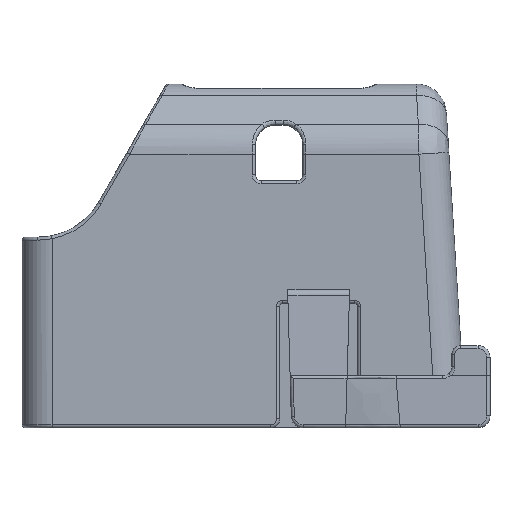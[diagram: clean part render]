
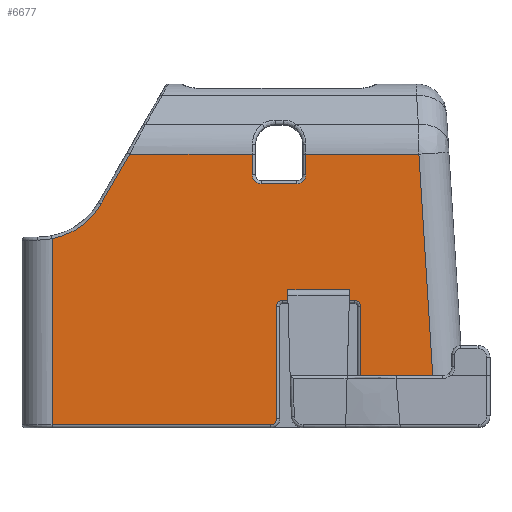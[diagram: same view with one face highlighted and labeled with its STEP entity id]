
A CAD part, left-side view. The second image highlights one B-rep face of the part: STEP entity #6677.
In plain terms, the highlighted planar face has unit normal (-1, 0, 0).
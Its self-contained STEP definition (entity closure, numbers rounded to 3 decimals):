
#21=PLANE('',#7149);
#565=LINE('',#10031,#1024);
#567=LINE('',#10138,#1026);
#568=LINE('',#10146,#1027);
#572=LINE('',#10219,#1031);
#573=LINE('',#10221,#1032);
#574=LINE('',#10225,#1033);
#575=LINE('',#10227,#1034);
#576=LINE('',#10231,#1035);
#577=LINE('',#10235,#1036);
#578=LINE('',#10237,#1037);
#579=LINE('',#10239,#1038);
#580=LINE('',#10241,#1039);
#581=LINE('',#10243,#1040);
#582=LINE('',#10247,#1041);
#583=LINE('',#10251,#1042);
#584=LINE('',#10253,#1043);
#585=LINE('',#10254,#1044);
#1024=VECTOR('',#7941,10.);
#1026=VECTOR('',#7969,10.);
#1027=VECTOR('',#7980,10.);
#1031=VECTOR('',#8000,10.);
#1032=VECTOR('',#8001,10.);
#1033=VECTOR('',#8004,10.);
#1034=VECTOR('',#8005,10.);
#1035=VECTOR('',#8008,10.);
#1036=VECTOR('',#8011,10.);
#1037=VECTOR('',#8012,10.);
#1038=VECTOR('',#8013,10.);
#1039=VECTOR('',#8014,10.);
#1040=VECTOR('',#8015,0.5);
#1041=VECTOR('',#8018,10.);
#1042=VECTOR('',#8021,10.);
#1043=VECTOR('',#8022,10.);
#1044=VECTOR('',#8023,10.);
#1631=FACE_OUTER_BOUND('',#2044,.T.);
#2044=EDGE_LOOP('',(#4598,#4599,#4600,#4601,#4602,#4603,#4604,#4605,#4606,
#4607,#4608,#4609,#4610,#4611,#4612,#4613,#4614,#4615,#4616,#4617,#4618,
#4619,#4620,#4621));
#2453=CIRCLE('',#7119,1.5);
#2469=CIRCLE('',#7140,1.5);
#2472=CIRCLE('',#7150,12.);
#2473=CIRCLE('',#7151,1.);
#2474=CIRCLE('',#7152,1.);
#2475=CIRCLE('',#7153,1.);
#2476=CIRCLE('',#7154,1.);
#2781=VERTEX_POINT('',#10019);
#2782=VERTEX_POINT('',#10021);
#2784=VERTEX_POINT('',#10027);
#2794=VERTEX_POINT('',#10128);
#2796=VERTEX_POINT('',#10134);
#2798=VERTEX_POINT('',#10140);
#2804=VERTEX_POINT('',#10218);
#2805=VERTEX_POINT('',#10220);
#2806=VERTEX_POINT('',#10222);
#2807=VERTEX_POINT('',#10224);
#2808=VERTEX_POINT('',#10226);
#2809=VERTEX_POINT('',#10228);
#2810=VERTEX_POINT('',#10230);
#2811=VERTEX_POINT('',#10232);
#2812=VERTEX_POINT('',#10234);
#2813=VERTEX_POINT('',#10236);
#2814=VERTEX_POINT('',#10238);
#2815=VERTEX_POINT('',#10240);
#2816=VERTEX_POINT('',#10242);
#2817=VERTEX_POINT('',#10244);
#2818=VERTEX_POINT('',#10246);
#2819=VERTEX_POINT('',#10248);
#2820=VERTEX_POINT('',#10250);
#2821=VERTEX_POINT('',#10252);
#3451=EDGE_CURVE('',#2781,#2782,#2453,.T.);
#3456=EDGE_CURVE('',#2782,#2784,#565,.T.);
#3472=EDGE_CURVE('',#2794,#2796,#567,.T.);
#3475=EDGE_CURVE('',#2796,#2798,#2469,.T.);
#3476=EDGE_CURVE('',#2798,#2781,#568,.T.);
#3486=EDGE_CURVE('',#2794,#2804,#572,.T.);
#3487=EDGE_CURVE('',#2805,#2804,#573,.T.);
#3488=EDGE_CURVE('',#2806,#2805,#2472,.T.);
#3489=EDGE_CURVE('',#2807,#2806,#574,.T.);
#3490=EDGE_CURVE('',#2808,#2807,#575,.T.);
#3491=EDGE_CURVE('',#2809,#2808,#2473,.T.);
#3492=EDGE_CURVE('',#2810,#2809,#576,.T.);
#3493=EDGE_CURVE('',#2811,#2810,#2474,.T.);
#3494=EDGE_CURVE('',#2812,#2811,#577,.T.);
#3495=EDGE_CURVE('',#2812,#2813,#578,.T.);
#3496=EDGE_CURVE('',#2813,#2814,#579,.T.);
#3497=EDGE_CURVE('',#2814,#2815,#580,.T.);
#3498=EDGE_CURVE('',#2815,#2816,#581,.T.);
#3499=EDGE_CURVE('',#2817,#2816,#2475,.T.);
#3500=EDGE_CURVE('',#2818,#2817,#582,.T.);
#3501=EDGE_CURVE('',#2819,#2818,#2476,.T.);
#3502=EDGE_CURVE('',#2820,#2819,#583,.T.);
#3503=EDGE_CURVE('',#2821,#2820,#584,.T.);
#3504=EDGE_CURVE('',#2821,#2784,#585,.T.);
#4598=ORIENTED_EDGE('',*,*,#3456,.F.);
#4599=ORIENTED_EDGE('',*,*,#3451,.F.);
#4600=ORIENTED_EDGE('',*,*,#3476,.F.);
#4601=ORIENTED_EDGE('',*,*,#3475,.F.);
#4602=ORIENTED_EDGE('',*,*,#3472,.F.);
#4603=ORIENTED_EDGE('',*,*,#3486,.T.);
#4604=ORIENTED_EDGE('',*,*,#3487,.F.);
#4605=ORIENTED_EDGE('',*,*,#3488,.F.);
#4606=ORIENTED_EDGE('',*,*,#3489,.F.);
#4607=ORIENTED_EDGE('',*,*,#3490,.F.);
#4608=ORIENTED_EDGE('',*,*,#3491,.F.);
#4609=ORIENTED_EDGE('',*,*,#3492,.F.);
#4610=ORIENTED_EDGE('',*,*,#3493,.F.);
#4611=ORIENTED_EDGE('',*,*,#3494,.F.);
#4612=ORIENTED_EDGE('',*,*,#3495,.T.);
#4613=ORIENTED_EDGE('',*,*,#3496,.T.);
#4614=ORIENTED_EDGE('',*,*,#3497,.T.);
#4615=ORIENTED_EDGE('',*,*,#3498,.T.);
#4616=ORIENTED_EDGE('',*,*,#3499,.F.);
#4617=ORIENTED_EDGE('',*,*,#3500,.F.);
#4618=ORIENTED_EDGE('',*,*,#3501,.F.);
#4619=ORIENTED_EDGE('',*,*,#3502,.F.);
#4620=ORIENTED_EDGE('',*,*,#3503,.F.);
#4621=ORIENTED_EDGE('',*,*,#3504,.T.);
#6677=ADVANCED_FACE('',(#1631),#21,.F.);
#7119=AXIS2_PLACEMENT_3D('',#10022,#7930,#7931);
#7140=AXIS2_PLACEMENT_3D('',#10144,#7976,#7977);
#7149=AXIS2_PLACEMENT_3D('',#10217,#7998,#7999);
#7150=AXIS2_PLACEMENT_3D('',#10223,#8002,#8003);
#7151=AXIS2_PLACEMENT_3D('',#10229,#8006,#8007);
#7152=AXIS2_PLACEMENT_3D('',#10233,#8009,#8010);
#7153=AXIS2_PLACEMENT_3D('',#10245,#8016,#8017);
#7154=AXIS2_PLACEMENT_3D('',#10249,#8019,#8020);
#7930=DIRECTION('center_axis',(-1.,0.,0.));
#7931=DIRECTION('ref_axis',(0.,-0.707,-0.707));
#7941=DIRECTION('',(0.,0.,1.));
#7969=DIRECTION('',(0.,0.,-1.));
#7976=DIRECTION('center_axis',(-1.,0.,0.));
#7977=DIRECTION('ref_axis',(0.,0.707,-0.707));
#7980=DIRECTION('',(0.,-1.,0.));
#7998=DIRECTION('center_axis',(1.,0.,0.));
#7999=DIRECTION('ref_axis',(0.,0.,-1.));
#8000=DIRECTION('',(0.,1.,0.));
#8001=DIRECTION('',(0.,-0.499,0.866));
#8002=DIRECTION('center_axis',(-1.,0.,0.));
#8003=DIRECTION('ref_axis',(0.,-0.583,-0.812));
#8004=DIRECTION('',(0.,0.,1.));
#8005=DIRECTION('',(0.,1.,0.));
#8006=DIRECTION('center_axis',(1.,0.,0.));
#8007=DIRECTION('ref_axis',(0.,-0.707,-0.707));
#8008=DIRECTION('',(0.,0.,-1.));
#8009=DIRECTION('center_axis',(-1.,0.,0.));
#8010=DIRECTION('ref_axis',(0.,0.707,0.707));
#8011=DIRECTION('',(0.,1.,0.));
#8012=DIRECTION('',(0.,0.,1.));
#8013=DIRECTION('',(0.,-1.,0.));
#8014=DIRECTION('',(0.,0.029,-1.));
#8015=DIRECTION('',(0.,-1.,0.));
#8016=DIRECTION('center_axis',(-1.,0.,0.));
#8017=DIRECTION('ref_axis',(0.,-0.707,0.707));
#8018=DIRECTION('',(0.,0.,1.));
#8019=DIRECTION('center_axis',(1.,0.,0.));
#8020=DIRECTION('ref_axis',(0.,0.707,-0.707));
#8021=DIRECTION('',(0.,1.,0.));
#8022=DIRECTION('',(0.,-0.062,-0.998));
#8023=DIRECTION('',(0.,1.,0.));
#10019=CARTESIAN_POINT('',(-118.44,-14.067,24.405));
#10021=CARTESIAN_POINT('',(-118.44,-15.567,25.905));
#10022=CARTESIAN_POINT('Origin',(-118.44,-14.067,25.905));
#10027=CARTESIAN_POINT('',(-118.44,-15.567,29.372));
#10031=CARTESIAN_POINT('',(-118.44,-15.567,16.859));
#10128=CARTESIAN_POINT('',(-118.44,-6.667,29.372));
#10134=CARTESIAN_POINT('',(-118.44,-6.667,25.905));
#10138=CARTESIAN_POINT('',(-118.44,-6.667,19.859));
#10140=CARTESIAN_POINT('',(-118.44,-8.167,24.405));
#10144=CARTESIAN_POINT('Origin',(-118.44,-8.167,25.905));
#10146=CARTESIAN_POINT('',(-118.44,-9.786,24.405));
#10217=CARTESIAN_POINT('Origin',(-118.44,-12.406,8.812));
#10218=CARTESIAN_POINT('',(-118.44,13.797,29.372));
#10219=CARTESIAN_POINT('',(-118.44,-56.546,29.372));
#10220=CARTESIAN_POINT('',(-118.44,18.591,21.057));
#10221=CARTESIAN_POINT('',(-118.44,11.452,33.44));
#10222=CARTESIAN_POINT('',(-118.44,26.734,15.264));
#10223=CARTESIAN_POINT('Origin',(-118.44,28.987,27.051));
#10224=CARTESIAN_POINT('',(-118.44,26.734,-15.759));
#10225=CARTESIAN_POINT('',(-118.44,26.734,14.575));
#10226=CARTESIAN_POINT('',(-118.44,-9.698,-15.759));
#10227=CARTESIAN_POINT('',(-118.44,-6.203,-15.759));
#10228=CARTESIAN_POINT('',(-118.44,-10.698,-14.759));
#10229=CARTESIAN_POINT('Origin',(-118.44,-9.698,-14.759));
#10230=CARTESIAN_POINT('',(-118.44,-10.698,3.973));
#10231=CARTESIAN_POINT('',(-118.44,-10.698,-3.723));
#10232=CARTESIAN_POINT('',(-118.44,-11.698,4.973));
#10233=CARTESIAN_POINT('Origin',(-118.44,-11.698,3.973));
#10234=CARTESIAN_POINT('',(-118.44,-12.586,4.973));
#10235=CARTESIAN_POINT('',(-118.44,-11.802,4.973));
#10236=CARTESIAN_POINT('',(-118.44,-12.586,6.789));
#10237=CARTESIAN_POINT('',(-118.44,-12.586,4.973));
#10238=CARTESIAN_POINT('',(-118.44,-22.869,6.789));
#10239=CARTESIAN_POINT('',(-118.44,-17.637,6.789));
#10240=CARTESIAN_POINT('',(-118.44,-22.816,4.973));
#10241=CARTESIAN_POINT('',(-118.44,-22.79,4.066));
#10242=CARTESIAN_POINT('',(-118.44,-23.704,4.973));
#10243=CARTESIAN_POINT('',(-118.44,-11.802,4.973));
#10244=CARTESIAN_POINT('',(-118.44,-24.704,3.973));
#10245=CARTESIAN_POINT('Origin',(-118.44,-23.704,3.973));
#10246=CARTESIAN_POINT('',(-118.44,-24.704,-14.759));
#10247=CARTESIAN_POINT('',(-118.44,-24.704,13.581));
#10248=CARTESIAN_POINT('',(-118.44,-25.704,-15.759));
#10249=CARTESIAN_POINT('Origin',(-118.44,-25.704,-14.759));
#10250=CARTESIAN_POINT('',(-118.44,-37.225,-15.759));
#10251=CARTESIAN_POINT('',(-118.44,-6.203,-15.759));
#10252=CARTESIAN_POINT('',(-118.44,-34.418,29.372));
#10253=CARTESIAN_POINT('',(-118.44,-36.441,-3.157));
#10254=CARTESIAN_POINT('',(-118.44,-56.546,29.372));
